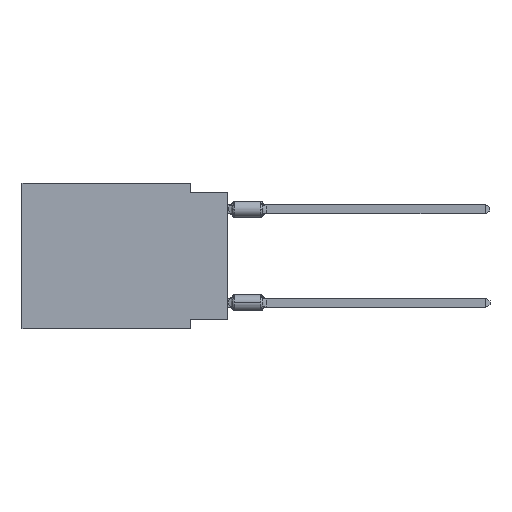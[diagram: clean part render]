
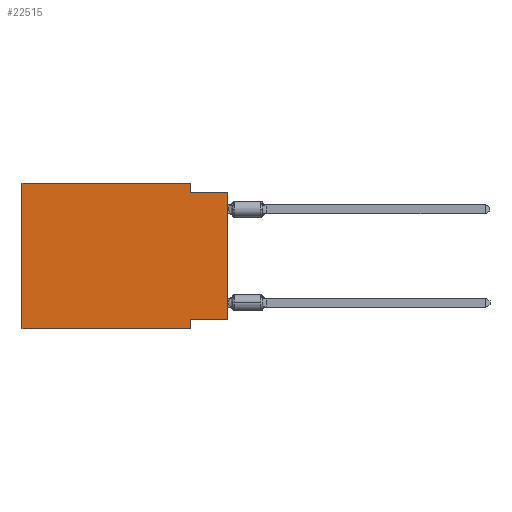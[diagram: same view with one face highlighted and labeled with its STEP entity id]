
A CAD part, left-side view. The second image highlights one B-rep face of the part: STEP entity #22515.
In plain terms, the highlighted planar face has unit normal (-1, 0, 0).
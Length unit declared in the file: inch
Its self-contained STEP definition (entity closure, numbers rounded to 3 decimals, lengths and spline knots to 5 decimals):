
#66 = DIRECTION ( 'NONE',  ( 0., -1., 0. ) ) ;
#514 = CARTESIAN_POINT ( 'NONE',  ( 0., 0.1, -0.365 ) ) ;
#886 = ORIENTED_EDGE ( 'NONE', *, *, #22319, .F. ) ;
#2421 = VERTEX_POINT ( 'NONE', #10926 ) ;
#2530 = EDGE_CURVE ( 'NONE', #19884, #2421, #23620, .T. ) ;
#3089 = DIRECTION ( 'NONE',  ( 0., 0., 1. ) ) ;
#3270 = CARTESIAN_POINT ( 'NONE',  ( 0., 0., 0. ) ) ;
#3445 = CARTESIAN_POINT ( 'NONE',  ( 0., 0.1, 0. ) ) ;
#3983 = VECTOR ( 'NONE', #66, 39.37008 ) ;
#3993 = CARTESIAN_POINT ( 'NONE',  ( 0., 0., -0.365 ) ) ;
#4618 = FACE_OUTER_BOUND ( 'NONE', #10908, .T. ) ;
#5341 = EDGE_CURVE ( 'NONE', #22369, #7252, #30324, .T. ) ;
#5460 = LINE ( 'NONE', #26428, #33449 ) ;
#6591 = EDGE_CURVE ( 'NONE', #21509, #7252, #5460, .T. ) ;
#7036 = CARTESIAN_POINT ( 'NONE',  ( 0., 0.55, 0. ) ) ;
#7252 = VERTEX_POINT ( 'NONE', #33698 ) ;
#8711 = DIRECTION ( 'NONE',  ( 0., -1., 0. ) ) ;
#8788 = LINE ( 'NONE', #3270, #19067 ) ;
#10771 = DIRECTION ( 'NONE',  ( 0., -1., 0. ) ) ;
#10827 = LINE ( 'NONE', #13754, #21828 ) ;
#10908 = EDGE_LOOP ( 'NONE', ( #31663, #16320, #886, #24262, #12539, #13056, #13569, #17972 ) ) ;
#10926 = CARTESIAN_POINT ( 'NONE',  ( 0., 0.1, 0. ) ) ;
#11047 = CARTESIAN_POINT ( 'NONE',  ( 0., 0., -0.365 ) ) ;
#11119 = VECTOR ( 'NONE', #14128, 39.37008 ) ;
#11718 = CARTESIAN_POINT ( 'NONE',  ( 0., 0.55, 0. ) ) ;
#12539 = ORIENTED_EDGE ( 'NONE', *, *, #22274, .F. ) ;
#12561 = VECTOR ( 'NONE', #32895, 39.37008 ) ;
#12860 = PLANE ( 'NONE',  #20146 ) ;
#13041 = VERTEX_POINT ( 'NONE', #33438 ) ;
#13056 = ORIENTED_EDGE ( 'NONE', *, *, #6591, .T. ) ;
#13569 = ORIENTED_EDGE ( 'NONE', *, *, #5341, .F. ) ;
#13754 = CARTESIAN_POINT ( 'NONE',  ( 0., 0.55, 0. ) ) ;
#14128 = DIRECTION ( 'NONE',  ( 0., 1., 0. ) ) ;
#15943 = VECTOR ( 'NONE', #8711, 39.37008 ) ;
#16320 = ORIENTED_EDGE ( 'NONE', *, *, #17970, .F. ) ;
#16489 = LINE ( 'NONE', #3445, #21806 ) ;
#17970 = EDGE_CURVE ( 'NONE', #13041, #32166, #21912, .T. ) ;
#17972 = ORIENTED_EDGE ( 'NONE', *, *, #30294, .F. ) ;
#18447 = VERTEX_POINT ( 'NONE', #11047 ) ;
#19067 = VECTOR ( 'NONE', #3089, 39.37008 ) ;
#19884 = VERTEX_POINT ( 'NONE', #11718 ) ;
#20146 = AXIS2_PLACEMENT_3D ( 'NONE', #7036, #28520, #26108 ) ;
#21509 = VERTEX_POINT ( 'NONE', #32393 ) ;
#21806 = VECTOR ( 'NONE', #29072, 39.37008 ) ;
#21828 = VECTOR ( 'NONE', #26481, 39.37008 ) ;
#21912 = LINE ( 'NONE', #32245, #15943 ) ;
#22253 = EDGE_CURVE ( 'NONE', #18447, #32166, #8788, .T. ) ;
#22274 = EDGE_CURVE ( 'NONE', #21509, #19884, #10827, .T. ) ;
#22319 = EDGE_CURVE ( 'NONE', #2421, #13041, #16489, .T. ) ;
#22369 = VERTEX_POINT ( 'NONE', #514 ) ;
#22515 = ADVANCED_FACE ( 'NONE', ( #4618 ), #12860, .F. ) ;
#23620 = LINE ( 'NONE', #28619, #3983 ) ;
#24262 = ORIENTED_EDGE ( 'NONE', *, *, #2530, .F. ) ;
#24987 = CARTESIAN_POINT ( 'NONE',  ( 0., 0.1, -0.39 ) ) ;
#26108 = DIRECTION ( 'NONE',  ( 0., 0., -1. ) ) ;
#26428 = CARTESIAN_POINT ( 'NONE',  ( 0., 0.55, -0.39 ) ) ;
#26481 = DIRECTION ( 'NONE',  ( 0., 0., 1. ) ) ;
#27714 = LINE ( 'NONE', #3993, #11119 ) ;
#28520 = DIRECTION ( 'NONE',  ( 1., 0., 0. ) ) ;
#28619 = CARTESIAN_POINT ( 'NONE',  ( 0., 0.55, 0. ) ) ;
#29072 = DIRECTION ( 'NONE',  ( 0., 0., -1. ) ) ;
#30294 = EDGE_CURVE ( 'NONE', #18447, #22369, #27714, .T. ) ;
#30324 = LINE ( 'NONE', #24987, #12561 ) ;
#31663 = ORIENTED_EDGE ( 'NONE', *, *, #22253, .T. ) ;
#31782 = CARTESIAN_POINT ( 'NONE',  ( 0., 0., -0.025 ) ) ;
#32166 = VERTEX_POINT ( 'NONE', #31782 ) ;
#32245 = CARTESIAN_POINT ( 'NONE',  ( 0., 0., -0.025 ) ) ;
#32393 = CARTESIAN_POINT ( 'NONE',  ( 0., 0.55, -0.39 ) ) ;
#32895 = DIRECTION ( 'NONE',  ( 0., 0., -1. ) ) ;
#33438 = CARTESIAN_POINT ( 'NONE',  ( 0., 0.1, -0.025 ) ) ;
#33449 = VECTOR ( 'NONE', #10771, 39.37008 ) ;
#33698 = CARTESIAN_POINT ( 'NONE',  ( 0., 0.1, -0.39 ) ) ;
